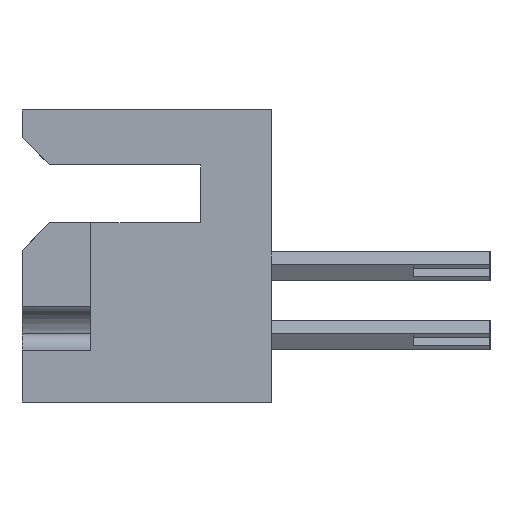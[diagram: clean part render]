
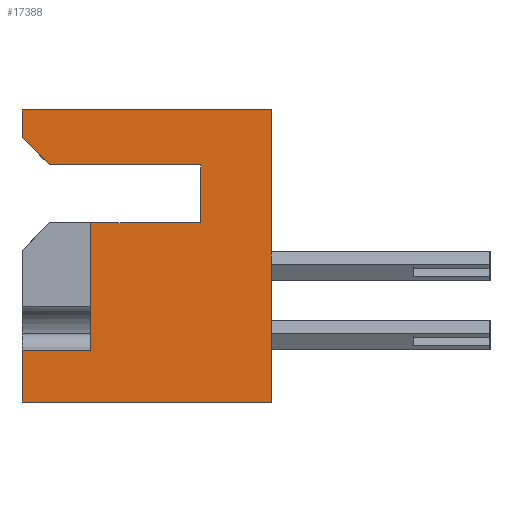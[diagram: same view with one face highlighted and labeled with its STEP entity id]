
A CAD part, left-side view. The second image highlights one B-rep face of the part: STEP entity #17388.
In plain terms, the highlighted planar face has unit normal (-1, 0, 0).
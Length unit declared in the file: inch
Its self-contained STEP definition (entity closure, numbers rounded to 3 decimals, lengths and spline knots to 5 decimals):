
#220 = DIRECTION ( 'NONE',  ( 0., -0.707, -0.707 ) ) ;
#319 = LINE ( 'NONE', #11933, #15185 ) ;
#582 = CARTESIAN_POINT ( 'NONE',  ( 0., 0.403, -0.1 ) ) ;
#590 = LINE ( 'NONE', #15155, #10612 ) ;
#2403 = VERTEX_POINT ( 'NONE', #582 ) ;
#2605 = VECTOR ( 'NONE', #24935, 39.37008 ) ;
#3374 = DIRECTION ( 'NONE',  ( 0., -1., 0. ) ) ;
#4332 = ORIENTED_EDGE ( 'NONE', *, *, #14638, .T. ) ;
#4492 = ORIENTED_EDGE ( 'NONE', *, *, #30202, .T. ) ;
#4699 = EDGE_CURVE ( 'NONE', #23562, #18039, #319, .T. ) ;
#4721 = CARTESIAN_POINT ( 'NONE',  ( 0., 0., -0.531 ) ) ;
#4941 = ORIENTED_EDGE ( 'NONE', *, *, #4699, .F. ) ;
#5004 = EDGE_CURVE ( 'NONE', #23566, #20794, #5460, .T. ) ;
#5024 = CARTESIAN_POINT ( 'NONE',  ( 0., 0., 0. ) ) ;
#5059 = CARTESIAN_POINT ( 'NONE',  ( 0., 0.403, -0.1 ) ) ;
#5460 = LINE ( 'NONE', #8246, #16651 ) ;
#5461 = DIRECTION ( 'NONE',  ( 0., -1., 0. ) ) ;
#5470 = VECTOR ( 'NONE', #30300, 39.37008 ) ;
#5610 = ORIENTED_EDGE ( 'NONE', *, *, #10243, .F. ) ;
#6128 = DIRECTION ( 'NONE',  ( 0., 1., 0. ) ) ;
#6313 = LINE ( 'NONE', #27144, #7068 ) ;
#6470 = ORIENTED_EDGE ( 'NONE', *, *, #24579, .T. ) ;
#6861 = CARTESIAN_POINT ( 'NONE',  ( 0., 0.128, -0.1 ) ) ;
#7068 = VECTOR ( 'NONE', #3374, 39.37008 ) ;
#7389 = LINE ( 'NONE', #15510, #15973 ) ;
#8246 = CARTESIAN_POINT ( 'NONE',  ( 0., 0., 0. ) ) ;
#9052 = VERTEX_POINT ( 'NONE', #22180 ) ;
#9186 = DIRECTION ( 'NONE',  ( 1., 0., 0. ) ) ;
#9542 = FACE_OUTER_BOUND ( 'NONE', #24477, .T. ) ;
#9795 = ORIENTED_EDGE ( 'NONE', *, *, #15579, .F. ) ;
#10243 = EDGE_CURVE ( 'NONE', #12025, #16677, #12639, .T. ) ;
#10612 = VECTOR ( 'NONE', #5461, 39.37008 ) ;
#10620 = DIRECTION ( 'NONE',  ( 0., 1., 0. ) ) ;
#11101 = VERTEX_POINT ( 'NONE', #16974 ) ;
#11702 = CARTESIAN_POINT ( 'NONE',  ( 0., 0.453, -0.05 ) ) ;
#11875 = VECTOR ( 'NONE', #220, 39.37008 ) ;
#11933 = CARTESIAN_POINT ( 'NONE',  ( 0., 0.453, 0. ) ) ;
#12025 = VERTEX_POINT ( 'NONE', #21676 ) ;
#12639 = LINE ( 'NONE', #20452, #20478 ) ;
#13273 = CARTESIAN_POINT ( 'NONE',  ( 0., 0.328, -0.205 ) ) ;
#13366 = DIRECTION ( 'NONE',  ( 0., 0., 1. ) ) ;
#13705 = DIRECTION ( 'NONE',  ( 0., 0., -1. ) ) ;
#14358 = DIRECTION ( 'NONE',  ( 0., 0., 1. ) ) ;
#14638 = EDGE_CURVE ( 'NONE', #12025, #18928, #26491, .T. ) ;
#15002 = ORIENTED_EDGE ( 'NONE', *, *, #5004, .T. ) ;
#15043 = VECTOR ( 'NONE', #30003, 39.37008 ) ;
#15155 = CARTESIAN_POINT ( 'NONE',  ( 0., 0.453, -0.531 ) ) ;
#15185 = VECTOR ( 'NONE', #14358, 39.37008 ) ;
#15510 = CARTESIAN_POINT ( 'NONE',  ( 0., 0.328, -0.437 ) ) ;
#15579 = EDGE_CURVE ( 'NONE', #18039, #20794, #6313, .T. ) ;
#15973 = VECTOR ( 'NONE', #6128, 39.37008 ) ;
#16178 = VECTOR ( 'NONE', #10620, 39.37008 ) ;
#16651 = VECTOR ( 'NONE', #29748, 39.37008 ) ;
#16677 = VERTEX_POINT ( 'NONE', #6861 ) ;
#16974 = CARTESIAN_POINT ( 'NONE',  ( 0., 0.453, -0.531 ) ) ;
#17388 = ADVANCED_FACE ( 'NONE', ( #9542 ), #27981, .F. ) ;
#17930 = CARTESIAN_POINT ( 'NONE',  ( 0., 0.128, -0.205 ) ) ;
#18039 = VERTEX_POINT ( 'NONE', #30627 ) ;
#18928 = VERTEX_POINT ( 'NONE', #13273 ) ;
#19216 = EDGE_CURVE ( 'NONE', #11101, #9052, #26968, .T. ) ;
#20336 = CARTESIAN_POINT ( 'NONE',  ( 0., 0.453, 0. ) ) ;
#20452 = CARTESIAN_POINT ( 'NONE',  ( 0., 0.128, -0.1 ) ) ;
#20478 = VECTOR ( 'NONE', #13366, 39.37008 ) ;
#20523 = VERTEX_POINT ( 'NONE', #27865 ) ;
#20794 = VERTEX_POINT ( 'NONE', #5024 ) ;
#20982 = EDGE_CURVE ( 'NONE', #16677, #2403, #30698, .T. ) ;
#21676 = CARTESIAN_POINT ( 'NONE',  ( 0., 0.128, -0.205 ) ) ;
#22141 = ORIENTED_EDGE ( 'NONE', *, *, #26238, .F. ) ;
#22180 = CARTESIAN_POINT ( 'NONE',  ( 0., 0.453, -0.437 ) ) ;
#22305 = LINE ( 'NONE', #5059, #11875 ) ;
#23189 = ORIENTED_EDGE ( 'NONE', *, *, #19216, .F. ) ;
#23497 = CARTESIAN_POINT ( 'NONE',  ( 0., 0.453, 0. ) ) ;
#23562 = VERTEX_POINT ( 'NONE', #11702 ) ;
#23566 = VERTEX_POINT ( 'NONE', #4721 ) ;
#24477 = EDGE_LOOP ( 'NONE', ( #6470, #23189, #29944, #15002, #9795, #4941, #4492, #29234, #5610, #4332, #22141 ) ) ;
#24579 = EDGE_CURVE ( 'NONE', #20523, #9052, #7389, .T. ) ;
#24911 = CARTESIAN_POINT ( 'NONE',  ( 0., 0.128, -0.1 ) ) ;
#24935 = DIRECTION ( 'NONE',  ( 0., 1., 0. ) ) ;
#25221 = CARTESIAN_POINT ( 'NONE',  ( 0., 0.328, -0.205 ) ) ;
#25250 = LINE ( 'NONE', #25221, #5470 ) ;
#26238 = EDGE_CURVE ( 'NONE', #20523, #18928, #25250, .T. ) ;
#26491 = LINE ( 'NONE', #17930, #2605 ) ;
#26968 = LINE ( 'NONE', #20336, #15043 ) ;
#27052 = EDGE_CURVE ( 'NONE', #11101, #23566, #590, .T. ) ;
#27144 = CARTESIAN_POINT ( 'NONE',  ( 0., 0.453, 0. ) ) ;
#27583 = AXIS2_PLACEMENT_3D ( 'NONE', #23497, #9186, #13705 ) ;
#27865 = CARTESIAN_POINT ( 'NONE',  ( 0., 0.328, -0.437 ) ) ;
#27981 = PLANE ( 'NONE',  #27583 ) ;
#29234 = ORIENTED_EDGE ( 'NONE', *, *, #20982, .F. ) ;
#29748 = DIRECTION ( 'NONE',  ( 0., 0., 1. ) ) ;
#29944 = ORIENTED_EDGE ( 'NONE', *, *, #27052, .T. ) ;
#30003 = DIRECTION ( 'NONE',  ( 0., 0., 1. ) ) ;
#30202 = EDGE_CURVE ( 'NONE', #23562, #2403, #22305, .T. ) ;
#30300 = DIRECTION ( 'NONE',  ( 0., 0., 1. ) ) ;
#30627 = CARTESIAN_POINT ( 'NONE',  ( 0., 0.453, 0. ) ) ;
#30698 = LINE ( 'NONE', #24911, #16178 ) ;
